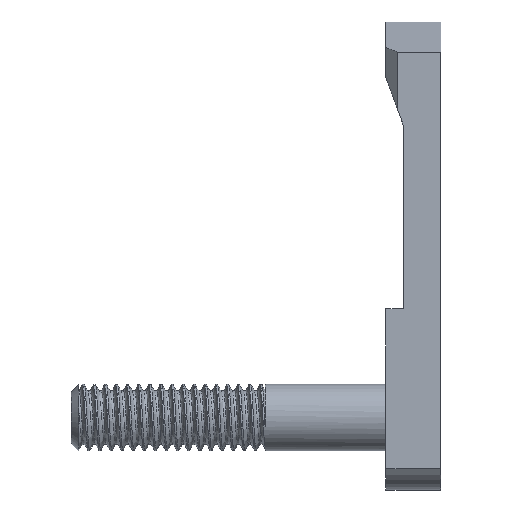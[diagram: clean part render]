
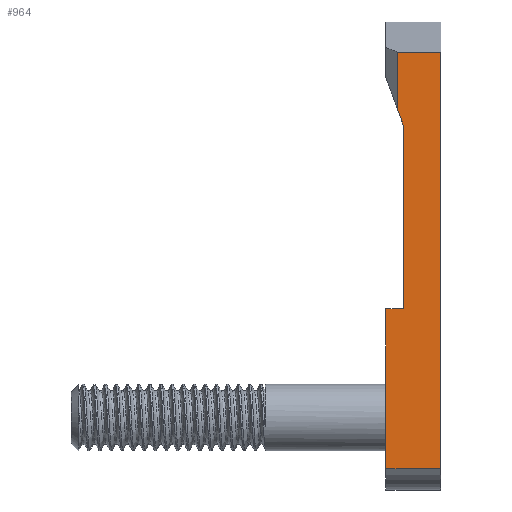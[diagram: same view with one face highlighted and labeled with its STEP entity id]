
A CAD part, front view. The second image highlights one B-rep face of the part: STEP entity #964.
In plain terms, the highlighted planar face has unit normal (0, -1, 0).
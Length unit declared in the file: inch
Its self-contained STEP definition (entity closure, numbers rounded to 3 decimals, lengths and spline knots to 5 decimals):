
#22=PLANE('',#1036);
#69=FACE_OUTER_BOUND('',#122,.T.);
#122=EDGE_LOOP('',(#747,#748,#749,#750,#751,#752,#753,#754));
#265=LINE('',#2492,#326);
#269=LINE('',#2501,#330);
#271=LINE('',#2505,#332);
#272=LINE('',#2507,#333);
#273=LINE('',#2509,#334);
#274=LINE('',#2511,#335);
#275=LINE('',#2513,#336);
#276=LINE('',#2514,#337);
#326=VECTOR('',#1178,0.3937);
#330=VECTOR('',#1186,0.3937);
#332=VECTOR('',#1190,0.3937);
#333=VECTOR('',#1191,0.3937);
#334=VECTOR('',#1192,0.3937);
#335=VECTOR('',#1193,0.3937);
#336=VECTOR('',#1194,0.3937);
#337=VECTOR('',#1195,0.3937);
#423=VERTEX_POINT('',#2484);
#426=VERTEX_POINT('',#2490);
#429=VERTEX_POINT('',#2500);
#430=VERTEX_POINT('',#2504);
#431=VERTEX_POINT('',#2506);
#432=VERTEX_POINT('',#2508);
#433=VERTEX_POINT('',#2510);
#434=VERTEX_POINT('',#2512);
#557=EDGE_CURVE('',#423,#426,#265,.T.);
#561=EDGE_CURVE('',#423,#429,#269,.T.);
#563=EDGE_CURVE('',#430,#426,#271,.T.);
#564=EDGE_CURVE('',#431,#430,#272,.T.);
#565=EDGE_CURVE('',#432,#431,#273,.T.);
#566=EDGE_CURVE('',#433,#432,#274,.T.);
#567=EDGE_CURVE('',#434,#433,#275,.T.);
#568=EDGE_CURVE('',#434,#429,#276,.T.);
#747=ORIENTED_EDGE('',*,*,#557,.T.);
#748=ORIENTED_EDGE('',*,*,#563,.F.);
#749=ORIENTED_EDGE('',*,*,#564,.F.);
#750=ORIENTED_EDGE('',*,*,#565,.F.);
#751=ORIENTED_EDGE('',*,*,#566,.F.);
#752=ORIENTED_EDGE('',*,*,#567,.F.);
#753=ORIENTED_EDGE('',*,*,#568,.T.);
#754=ORIENTED_EDGE('',*,*,#561,.F.);
#964=ADVANCED_FACE('',(#69),#22,.F.);
#1036=AXIS2_PLACEMENT_3D('',#2503,#1188,#1189);
#1178=DIRECTION('',(0.342,0.,-0.94));
#1186=DIRECTION('',(0.,0.,1.));
#1188=DIRECTION('center_axis',(0.,1.,0.));
#1189=DIRECTION('ref_axis',(0.,0.,-1.));
#1190=DIRECTION('',(0.,0.,1.));
#1191=DIRECTION('',(1.,0.,0.));
#1192=DIRECTION('',(0.,0.,1.));
#1193=DIRECTION('',(-1.,0.,0.));
#1194=DIRECTION('',(0.,0.,-1.));
#1195=DIRECTION('',(-1.,0.,0.));
#2484=CARTESIAN_POINT('',(0.032,-0.105,0.95171));
#2490=CARTESIAN_POINT('',(0.049,-0.105,0.905));
#2492=CARTESIAN_POINT('',(0.02215,-0.105,0.97876));
#2500=CARTESIAN_POINT('',(0.032,-0.105,1.11029));
#2501=CARTESIAN_POINT('',(0.032,-0.105,1.00589));
#2503=CARTESIAN_POINT('Origin',(0.154,-0.105,1.11029));
#2504=CARTESIAN_POINT('',(0.049,-0.105,0.388));
#2505=CARTESIAN_POINT('',(0.049,-0.105,0.98314));
#2506=CARTESIAN_POINT('',(0.,-0.105,0.388));
#2507=CARTESIAN_POINT('',(0.077,-0.105,0.388));
#2508=CARTESIAN_POINT('',(0.,-0.105,-0.06212));
#2509=CARTESIAN_POINT('',(0.,-0.105,0.85564));
#2510=CARTESIAN_POINT('',(0.154,-0.105,-0.06212));
#2511=CARTESIAN_POINT('',(0.,-0.105,-0.06212));
#2512=CARTESIAN_POINT('',(0.154,-0.105,1.11029));
#2513=CARTESIAN_POINT('',(0.154,-0.105,0.85564));
#2514=CARTESIAN_POINT('',(0.154,-0.105,1.11029));
